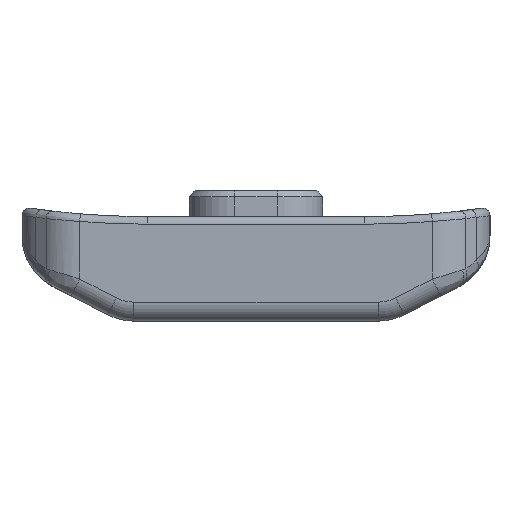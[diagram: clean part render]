
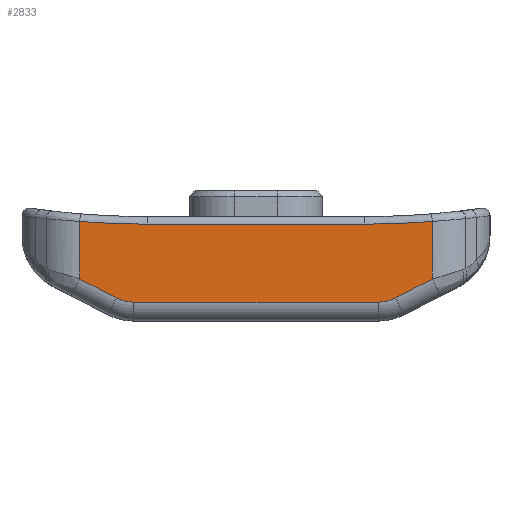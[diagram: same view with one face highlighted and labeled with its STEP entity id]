
A CAD part, front view. The second image highlights one B-rep face of the part: STEP entity #2833.
In plain terms, the highlighted planar face has unit normal (0, -1, 0).
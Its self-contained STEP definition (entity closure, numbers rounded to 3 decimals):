
#254=CIRCLE('',#2980,2.);
#272=CIRCLE('',#3008,2.);
#289=CIRCLE('',#3042,43.691);
#356=CIRCLE('',#3151,43.691);
#563=FACE_OUTER_BOUND('',#759,.T.);
#759=EDGE_LOOP('',(#2542,#2543,#2544,#2545,#2546,#2547,#2548,#2549,#2550,
#2551));
#895=LINE('',#4446,#1071);
#909=LINE('',#4507,#1085);
#939=LINE('',#5112,#1115);
#943=LINE('',#5552,#1119);
#944=LINE('',#5647,#1120);
#945=LINE('',#5649,#1121);
#1071=VECTOR('',#3589,10.);
#1085=VECTOR('',#3653,10.);
#1115=VECTOR('',#3949,10.);
#1119=VECTOR('',#4031,10.);
#1120=VECTOR('',#4042,10.);
#1121=VECTOR('',#4045,10.);
#1232=VERTEX_POINT('',#4422);
#1233=VERTEX_POINT('',#4424);
#1240=VERTEX_POINT('',#4444);
#1254=VERTEX_POINT('',#4482);
#1257=VERTEX_POINT('',#4487);
#1262=VERTEX_POINT('',#4506);
#1290=VERTEX_POINT('',#4724);
#1291=VERTEX_POINT('',#4731);
#1348=VERTEX_POINT('',#5110);
#1349=VERTEX_POINT('',#5114);
#1539=EDGE_CURVE('',#1232,#1233,#254,.T.);
#1550=EDGE_CURVE('',#1240,#1232,#895,.T.);
#1571=EDGE_CURVE('',#1257,#1254,#272,.T.);
#1580=EDGE_CURVE('',#1254,#1262,#909,.T.);
#1621=EDGE_CURVE('',#1291,#1290,#289,.T.);
#1723=EDGE_CURVE('',#1348,#1291,#939,.T.);
#1725=EDGE_CURVE('',#1349,#1348,#356,.T.);
#1768=EDGE_CURVE('',#1233,#1257,#943,.T.);
#1774=EDGE_CURVE('',#1262,#1349,#944,.T.);
#1775=EDGE_CURVE('',#1290,#1240,#945,.T.);
#2542=ORIENTED_EDGE('',*,*,#1539,.F.);
#2543=ORIENTED_EDGE('',*,*,#1550,.F.);
#2544=ORIENTED_EDGE('',*,*,#1775,.F.);
#2545=ORIENTED_EDGE('',*,*,#1621,.F.);
#2546=ORIENTED_EDGE('',*,*,#1723,.F.);
#2547=ORIENTED_EDGE('',*,*,#1725,.F.);
#2548=ORIENTED_EDGE('',*,*,#1774,.F.);
#2549=ORIENTED_EDGE('',*,*,#1580,.F.);
#2550=ORIENTED_EDGE('',*,*,#1571,.F.);
#2551=ORIENTED_EDGE('',*,*,#1768,.F.);
#2655=PLANE('',#3193);
#2833=ADVANCED_FACE('',(#563),#2655,.T.);
#2980=AXIS2_PLACEMENT_3D('',#4425,#3564,#3565);
#3008=AXIS2_PLACEMENT_3D('',#4489,#3632,#3633);
#3042=AXIS2_PLACEMENT_3D('',#4733,#3710,#3711);
#3151=AXIS2_PLACEMENT_3D('',#5116,#3954,#3955);
#3193=AXIS2_PLACEMENT_3D('',#5648,#4043,#4044);
#3564=DIRECTION('center_axis',(0.,1.,0.));
#3565=DIRECTION('ref_axis',(0.235,0.,-0.972));
#3589=DIRECTION('',(-0.889,0.,-0.457));
#3632=DIRECTION('center_axis',(0.,1.,0.));
#3633=DIRECTION('ref_axis',(-0.235,0.,-0.972));
#3653=DIRECTION('',(-0.889,0.,0.457));
#3710=DIRECTION('center_axis',(0.,-1.,0.));
#3711=DIRECTION('ref_axis',(0.041,0.,-0.999));
#3949=DIRECTION('',(1.,0.,0.));
#3954=DIRECTION('center_axis',(0.,-1.,0.));
#3955=DIRECTION('ref_axis',(-0.041,0.,-0.999));
#4031=DIRECTION('',(-1.,0.,0.));
#4042=DIRECTION('',(0.,0.,1.));
#4043=DIRECTION('center_axis',(0.,-1.,0.));
#4044=DIRECTION('ref_axis',(0.,0.,-1.));
#4045=DIRECTION('',(0.,0.,-1.));
#4422=CARTESIAN_POINT('',(-112.665,-75.5,-7.079));
#4424=CARTESIAN_POINT('',(-113.579,-75.5,-7.3));
#4425=CARTESIAN_POINT('Origin',(-113.579,-75.5,-5.3));
#4444=CARTESIAN_POINT('',(-110.736,-75.5,-6.088));
#4446=CARTESIAN_POINT('',(-115.444,-75.5,-8.507));
#4482=CARTESIAN_POINT('',(-127.335,-75.5,-7.079));
#4487=CARTESIAN_POINT('',(-126.421,-75.5,-7.3));
#4489=CARTESIAN_POINT('Origin',(-126.421,-75.5,-5.3));
#4506=CARTESIAN_POINT('',(-129.264,-75.5,-6.088));
#4507=CARTESIAN_POINT('',(-127.232,-75.5,-7.132));
#4724=CARTESIAN_POINT('',(-110.736,-75.5,-3.055));
#4731=CARTESIAN_POINT('',(-114.287,-75.5,-3.2));
#4733=CARTESIAN_POINT('Origin',(-114.287,-75.5,40.491));
#5110=CARTESIAN_POINT('',(-125.713,-75.5,-3.2));
#5112=CARTESIAN_POINT('',(-120.,-75.5,-3.2));
#5114=CARTESIAN_POINT('',(-129.264,-75.5,-3.055));
#5116=CARTESIAN_POINT('Origin',(-125.713,-75.5,40.491));
#5552=CARTESIAN_POINT('',(-126.25,-75.5,-7.3));
#5647=CARTESIAN_POINT('',(-129.264,-75.5,-4.368));
#5648=CARTESIAN_POINT('Origin',(-120.,-75.5,-4.89));
#5649=CARTESIAN_POINT('',(-110.736,-75.5,-4.368));
